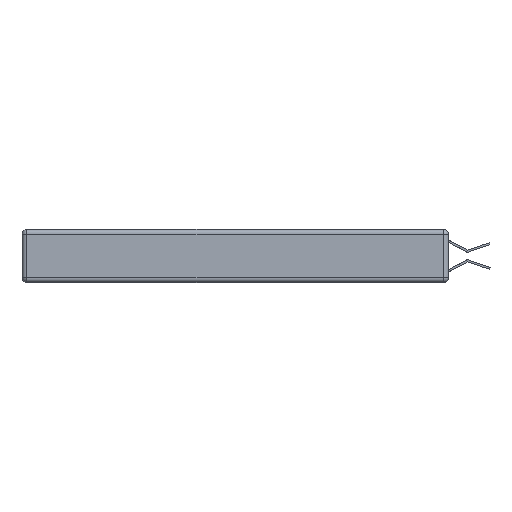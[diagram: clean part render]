
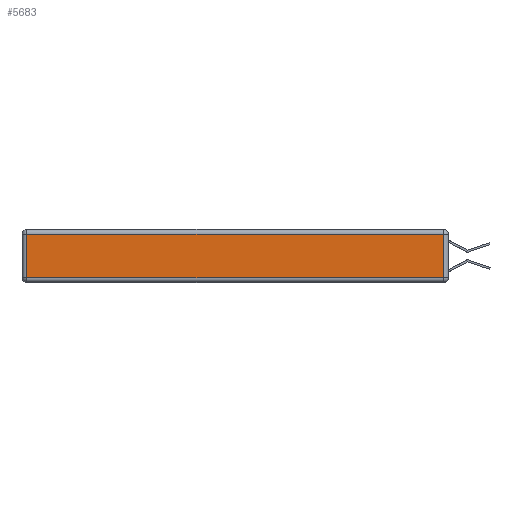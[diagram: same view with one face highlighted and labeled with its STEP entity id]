
A CAD part, left-side view. The second image highlights one B-rep face of the part: STEP entity #5683.
In plain terms, the highlighted planar face has unit normal (-1, 0, 0).
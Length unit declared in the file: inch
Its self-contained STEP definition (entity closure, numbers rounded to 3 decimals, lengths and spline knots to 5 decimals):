
#11 = VERTEX_POINT ( 'NONE', #9929 ) ;
#463 = LINE ( 'NONE', #3914, #11866 ) ;
#1117 = FACE_OUTER_BOUND ( 'NONE', #13871, .T. ) ;
#1441 = CARTESIAN_POINT ( 'NONE',  ( 0., 2.72, -0.313 ) ) ;
#2285 = VERTEX_POINT ( 'NONE', #14605 ) ;
#2342 = DIRECTION ( 'NONE',  ( 0., -1., 0. ) ) ;
#2803 = ORIENTED_EDGE ( 'NONE', *, *, #5626, .T. ) ;
#2864 = LINE ( 'NONE', #3179, #11875 ) ;
#3179 = CARTESIAN_POINT ( 'NONE',  ( 0., 2.72, -0.343 ) ) ;
#3499 = LINE ( 'NONE', #4846, #15208 ) ;
#3537 = DIRECTION ( 'NONE',  ( -1., 0., 0. ) ) ;
#3914 = CARTESIAN_POINT ( 'NONE',  ( 0., 0.03, -0.343 ) ) ;
#4228 = ORIENTED_EDGE ( 'NONE', *, *, #9988, .T. ) ;
#4805 = EDGE_CURVE ( 'NONE', #10725, #11, #463, .T. ) ;
#4846 = CARTESIAN_POINT ( 'NONE',  ( 0., 0., -0.313 ) ) ;
#4934 = ORIENTED_EDGE ( 'NONE', *, *, #15187, .T. ) ;
#5626 = EDGE_CURVE ( 'NONE', #11, #2285, #8129, .T. ) ;
#5683 = ADVANCED_FACE ( 'NONE', ( #1117 ), #13034, .T. ) ;
#5731 = DIRECTION ( 'NONE',  ( 0., 0., 1. ) ) ;
#5752 = VERTEX_POINT ( 'NONE', #1441 ) ;
#6337 = DIRECTION ( 'NONE',  ( 0., 0., 1. ) ) ;
#6900 = DIRECTION ( 'NONE',  ( 0., 1., 0. ) ) ;
#7450 = AXIS2_PLACEMENT_3D ( 'NONE', #8292, #3537, #5731 ) ;
#7924 = DIRECTION ( 'NONE',  ( 0., 0., -1. ) ) ;
#8129 = LINE ( 'NONE', #8215, #9171 ) ;
#8198 = ORIENTED_EDGE ( 'NONE', *, *, #4805, .T. ) ;
#8215 = CARTESIAN_POINT ( 'NONE',  ( 0., 2.75, -0.03 ) ) ;
#8292 = CARTESIAN_POINT ( 'NONE',  ( 0., 0., -0.343 ) ) ;
#9171 = VECTOR ( 'NONE', #6900, 39.37008 ) ;
#9929 = CARTESIAN_POINT ( 'NONE',  ( 0., 0.03, -0.03 ) ) ;
#9988 = EDGE_CURVE ( 'NONE', #5752, #10725, #3499, .T. ) ;
#10398 = CARTESIAN_POINT ( 'NONE',  ( 0., 0.03, -0.313 ) ) ;
#10725 = VERTEX_POINT ( 'NONE', #10398 ) ;
#11866 = VECTOR ( 'NONE', #6337, 39.37008 ) ;
#11875 = VECTOR ( 'NONE', #7924, 39.37008 ) ;
#13034 = PLANE ( 'NONE',  #7450 ) ;
#13871 = EDGE_LOOP ( 'NONE', ( #4228, #8198, #2803, #4934 ) ) ;
#14605 = CARTESIAN_POINT ( 'NONE',  ( 0., 2.72, -0.03 ) ) ;
#15187 = EDGE_CURVE ( 'NONE', #2285, #5752, #2864, .T. ) ;
#15208 = VECTOR ( 'NONE', #2342, 39.37008 ) ;
